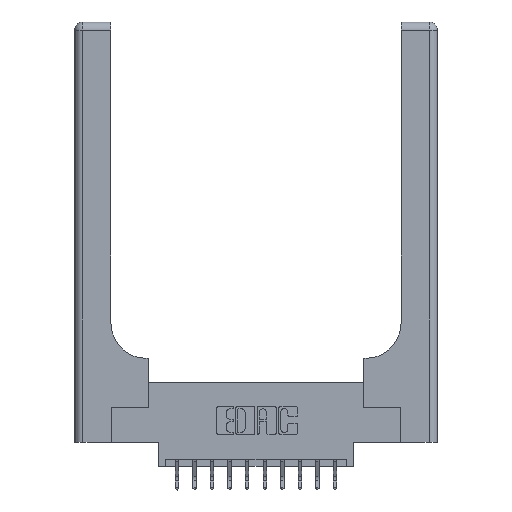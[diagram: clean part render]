
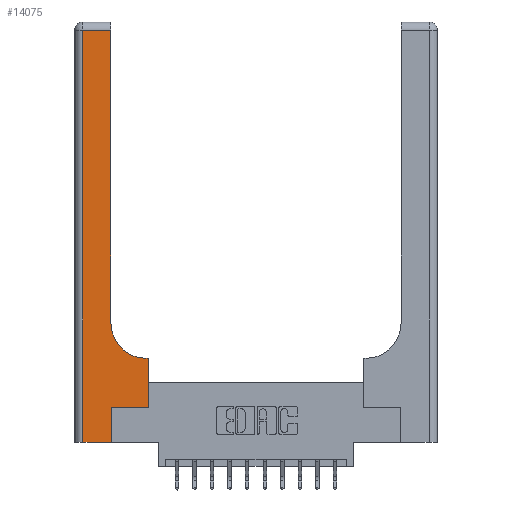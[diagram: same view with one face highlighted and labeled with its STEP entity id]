
A CAD part, top view. The second image highlights one B-rep face of the part: STEP entity #14075.
In plain terms, the highlighted planar face has unit normal (0, 0, 1).
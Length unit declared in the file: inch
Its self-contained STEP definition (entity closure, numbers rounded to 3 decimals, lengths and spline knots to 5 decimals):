
#476 = CARTESIAN_POINT ( 'NONE',  ( 0.26, 3., 0.37 ) ) ;
#522 = DIRECTION ( 'NONE',  ( -1., 0., 0. ) ) ;
#662 = VERTEX_POINT ( 'NONE', #5505 ) ;
#664 = VERTEX_POINT ( 'NONE', #5544 ) ;
#714 = DIRECTION ( 'NONE',  ( 0., 1., 0. ) ) ;
#847 = AXIS2_PLACEMENT_3D ( 'NONE', #7413, #1030, #9941 ) ;
#854 = LINE ( 'NONE', #476, #4257 ) ;
#1030 = DIRECTION ( 'NONE',  ( 0., 0., -1. ) ) ;
#1105 = EDGE_CURVE ( 'NONE', #15557, #2073, #5420, .T. ) ;
#1458 = DIRECTION ( 'NONE',  ( 1., 0., 0. ) ) ;
#1477 = DIRECTION ( 'NONE',  ( 0., 0., -1. ) ) ;
#1497 = CARTESIAN_POINT ( 'NONE',  ( 0.51, 0.85, 0.37 ) ) ;
#1598 = ORIENTED_EDGE ( 'NONE', *, *, #7579, .T. ) ;
#1678 = EDGE_CURVE ( 'NONE', #10749, #15557, #13895, .T. ) ;
#2073 = VERTEX_POINT ( 'NONE', #14961 ) ;
#2131 = VECTOR ( 'NONE', #522, 39.37008 ) ;
#2161 = EDGE_CURVE ( 'NONE', #6838, #13447, #7552, .T. ) ;
#2245 = ORIENTED_EDGE ( 'NONE', *, *, #9690, .T. ) ;
#2415 = EDGE_LOOP ( 'NONE', ( #12567, #2564, #1598, #3986, #6080, #2245, #12828, #9441, #14931 ) ) ;
#2437 = CARTESIAN_POINT ( 'NONE',  ( 0.06, 2.94, 0.37 ) ) ;
#2564 = ORIENTED_EDGE ( 'NONE', *, *, #10522, .T. ) ;
#2590 = CARTESIAN_POINT ( 'NONE',  ( 0.06, 3., 0.37 ) ) ;
#3039 = CARTESIAN_POINT ( 'NONE',  ( 0.265, 0.25, 0.37 ) ) ;
#3761 = VECTOR ( 'NONE', #8061, 39.37008 ) ;
#3986 = ORIENTED_EDGE ( 'NONE', *, *, #5995, .T. ) ;
#4206 = VECTOR ( 'NONE', #14036, 39.37008 ) ;
#4257 = VECTOR ( 'NONE', #10667, 39.37008 ) ;
#5420 = CIRCLE ( 'NONE', #11513, 0.25 ) ;
#5505 = CARTESIAN_POINT ( 'NONE',  ( 0.528, 0.25, 0.37 ) ) ;
#5544 = CARTESIAN_POINT ( 'NONE',  ( 0.26, 2.94, 0.37 ) ) ;
#5995 = EDGE_CURVE ( 'NONE', #12140, #6838, #15518, .T. ) ;
#6080 = ORIENTED_EDGE ( 'NONE', *, *, #2161, .T. ) ;
#6119 = LINE ( 'NONE', #15816, #16134 ) ;
#6180 = VECTOR ( 'NONE', #11945, 39.37008 ) ;
#6581 = LINE ( 'NONE', #3039, #6180 ) ;
#6838 = VERTEX_POINT ( 'NONE', #10331 ) ;
#7214 = CARTESIAN_POINT ( 'NONE',  ( 0., 0., 0.37 ) ) ;
#7413 = CARTESIAN_POINT ( 'NONE',  ( 0., 3., 0.37 ) ) ;
#7552 = LINE ( 'NONE', #7595, #11323 ) ;
#7579 = EDGE_CURVE ( 'NONE', #15426, #12140, #7602, .T. ) ;
#7595 = CARTESIAN_POINT ( 'NONE',  ( 0.265, 0., 0.37 ) ) ;
#7602 = LINE ( 'NONE', #2590, #4206 ) ;
#8061 = DIRECTION ( 'NONE',  ( -1., 0., 0. ) ) ;
#8834 = VECTOR ( 'NONE', #16038, 39.37008 ) ;
#9441 = ORIENTED_EDGE ( 'NONE', *, *, #1678, .T. ) ;
#9690 = EDGE_CURVE ( 'NONE', #13447, #662, #6581, .T. ) ;
#9941 = DIRECTION ( 'NONE',  ( -1., 0., 0. ) ) ;
#10331 = CARTESIAN_POINT ( 'NONE',  ( 0.265, 0., 0.37 ) ) ;
#10522 = EDGE_CURVE ( 'NONE', #664, #15426, #11904, .T. ) ;
#10667 = DIRECTION ( 'NONE',  ( 0., 1., 0. ) ) ;
#10749 = VERTEX_POINT ( 'NONE', #11048 ) ;
#11048 = CARTESIAN_POINT ( 'NONE',  ( 0.528, 0.6, 0.37 ) ) ;
#11323 = VECTOR ( 'NONE', #16360, 39.37008 ) ;
#11480 = FACE_OUTER_BOUND ( 'NONE', #2415, .T. ) ;
#11513 = AXIS2_PLACEMENT_3D ( 'NONE', #1497, #1477, #1458 ) ;
#11683 = EDGE_CURVE ( 'NONE', #662, #10749, #6119, .T. ) ;
#11904 = LINE ( 'NONE', #13227, #2131 ) ;
#11945 = DIRECTION ( 'NONE',  ( 1., 0., 0. ) ) ;
#12140 = VERTEX_POINT ( 'NONE', #14614 ) ;
#12567 = ORIENTED_EDGE ( 'NONE', *, *, #16067, .T. ) ;
#12828 = ORIENTED_EDGE ( 'NONE', *, *, #11683, .T. ) ;
#13089 = CARTESIAN_POINT ( 'NONE',  ( 0.51, 0.6, 0.37 ) ) ;
#13227 = CARTESIAN_POINT ( 'NONE',  ( 0., 2.94, 0.37 ) ) ;
#13447 = VERTEX_POINT ( 'NONE', #13679 ) ;
#13679 = CARTESIAN_POINT ( 'NONE',  ( 0.265, 0.25, 0.37 ) ) ;
#13895 = LINE ( 'NONE', #14344, #3761 ) ;
#14036 = DIRECTION ( 'NONE',  ( 0., -1., 0. ) ) ;
#14075 = ADVANCED_FACE ( 'NONE', ( #11480 ), #16184, .F. ) ;
#14344 = CARTESIAN_POINT ( 'NONE',  ( 0.26, 0.6, 0.37 ) ) ;
#14614 = CARTESIAN_POINT ( 'NONE',  ( 0.06, 0., 0.37 ) ) ;
#14931 = ORIENTED_EDGE ( 'NONE', *, *, #1105, .T. ) ;
#14961 = CARTESIAN_POINT ( 'NONE',  ( 0.26, 0.85, 0.37 ) ) ;
#15426 = VERTEX_POINT ( 'NONE', #2437 ) ;
#15518 = LINE ( 'NONE', #7214, #8834 ) ;
#15557 = VERTEX_POINT ( 'NONE', #13089 ) ;
#15816 = CARTESIAN_POINT ( 'NONE',  ( 0.528, 0.25, 0.37 ) ) ;
#16038 = DIRECTION ( 'NONE',  ( 1., 0., 0. ) ) ;
#16067 = EDGE_CURVE ( 'NONE', #2073, #664, #854, .T. ) ;
#16134 = VECTOR ( 'NONE', #714, 39.37008 ) ;
#16184 = PLANE ( 'NONE',  #847 ) ;
#16360 = DIRECTION ( 'NONE',  ( 0., 1., 0. ) ) ;
